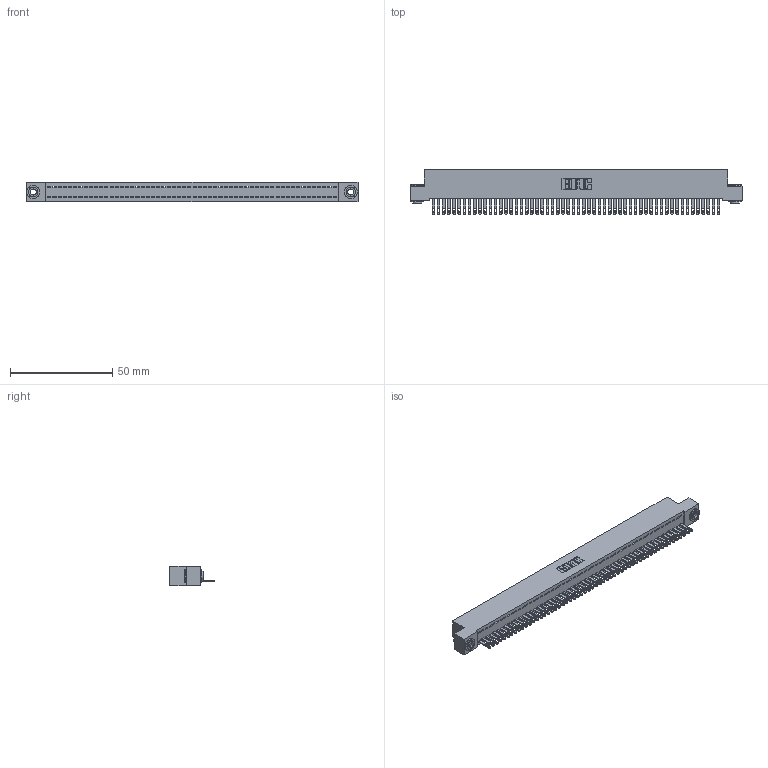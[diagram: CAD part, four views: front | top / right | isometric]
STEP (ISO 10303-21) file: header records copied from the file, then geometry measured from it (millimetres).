
FILE_DESCRIPTION (( 'STEP AP203' ), '1' );
FILE_NAME ('892-056-500-103.STEP', '2020-09-21T18:37:53', ( '' ), ( '' ), 'SwSTEP 2.0', 'SolidWorks 2020', '' );
FILE_SCHEMA (( 'CONFIG_CONTROL_DESIGN' ));
Length unit declared in the file: inch
Products named in the file (4): 892-056-500-103; 342-250-002_345-250-002-102; 842 Part_.156 TH; 345-292-001_345-293-100
Assembly tree (59 placements, depth 2):
  892-056-500-103
    842 Part_.156 TH
    345-292-001_345-293-100  x56
    342-250-002_345-250-002-102  x2
Bounding box: 162.56 x 21.85 x 9.4 mm (x, y, z)
Volume: 14362.3 mm3; surface area: 21688.2 mm2
Topology: 59 solids, 59 shells, 3172 faces, 9783 edges, 6518 vertices
Faces by surface type: plane 2092, cylinder 1072, cone 8
Entity records: 32872 total; most frequent: CARTESIAN_POINT 5645, ORIENTED_EDGE 5630, DIRECTION 4769, EDGE_CURVE 2815, VECTOR 2659, LINE 2659, VERTEX_POINT 1874, AXIS2_PLACEMENT_3D 1055
